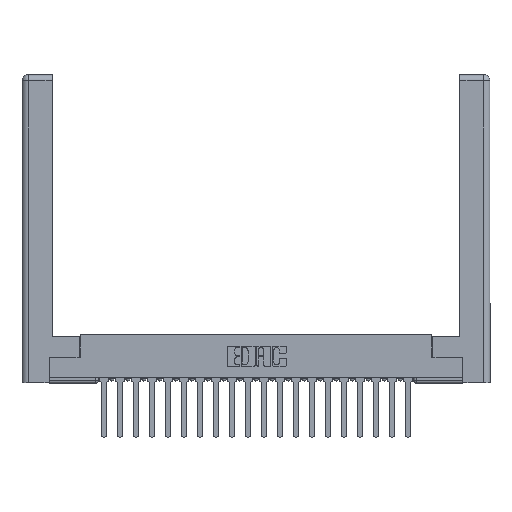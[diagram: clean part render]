
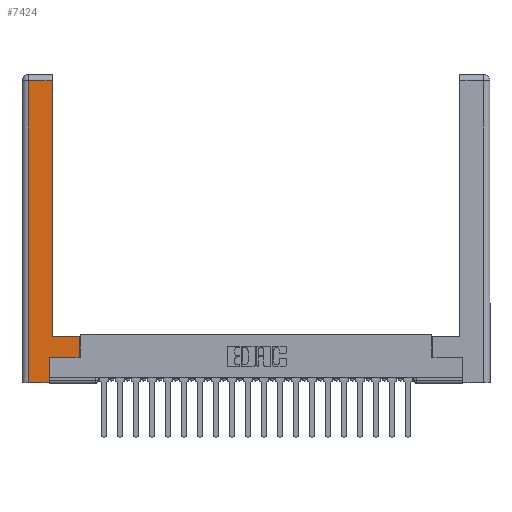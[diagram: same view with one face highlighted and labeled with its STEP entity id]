
A CAD part, top view. The second image highlights one B-rep face of the part: STEP entity #7424.
In plain terms, the highlighted planar face has unit normal (0, 0, 1).
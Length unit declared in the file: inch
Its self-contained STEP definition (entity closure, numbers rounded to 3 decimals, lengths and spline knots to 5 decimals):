
#573 = EDGE_CURVE ( 'NONE', #22322, #12661, #9282, .T. ) ;
#1147 = CARTESIAN_POINT ( 'NONE',  ( 0.0615, 2.94, 0. ) ) ;
#1283 = DIRECTION ( 'NONE',  ( -1., 0., 0. ) ) ;
#1405 = ORIENTED_EDGE ( 'NONE', *, *, #15285, .T. ) ;
#1590 = ORIENTED_EDGE ( 'NONE', *, *, #15119, .T. ) ;
#1652 = VERTEX_POINT ( 'NONE', #21168 ) ;
#1779 = AXIS2_PLACEMENT_3D ( 'NONE', #21097, #19411, #1968 ) ;
#1882 = EDGE_LOOP ( 'NONE', ( #5170, #1590, #4736, #4244, #5856, #15003, #1405, #17423 ) ) ;
#1891 = PLANE ( 'NONE',  #1779 ) ;
#1968 = DIRECTION ( 'NONE',  ( -1., 0., 0. ) ) ;
#2140 = CARTESIAN_POINT ( 'NONE',  ( 0.565, 0.45, 0. ) ) ;
#2605 = DIRECTION ( 'NONE',  ( 1., 0., 0. ) ) ;
#2776 = VECTOR ( 'NONE', #9026, 39.37008 ) ;
#3618 = CARTESIAN_POINT ( 'NONE',  ( 0.565, 0.245, 0. ) ) ;
#4244 = ORIENTED_EDGE ( 'NONE', *, *, #573, .T. ) ;
#4407 = FACE_OUTER_BOUND ( 'NONE', #1882, .T. ) ;
#4505 = VERTEX_POINT ( 'NONE', #8392 ) ;
#4682 = DIRECTION ( 'NONE',  ( 0., 1., 0. ) ) ;
#4711 = EDGE_CURVE ( 'NONE', #1652, #10802, #8016, .T. ) ;
#4736 = ORIENTED_EDGE ( 'NONE', *, *, #14170, .T. ) ;
#4840 = VECTOR ( 'NONE', #1283, 39.37008 ) ;
#5170 = ORIENTED_EDGE ( 'NONE', *, *, #14930, .T. ) ;
#5437 = CARTESIAN_POINT ( 'NONE',  ( 0.0615, 0., 0. ) ) ;
#5856 = ORIENTED_EDGE ( 'NONE', *, *, #10241, .T. ) ;
#6187 = CARTESIAN_POINT ( 'NONE',  ( 0.295, 0.45, 0. ) ) ;
#6730 = CARTESIAN_POINT ( 'NONE',  ( 0.565, 0.245, 0. ) ) ;
#7178 = VECTOR ( 'NONE', #12036, 39.37008 ) ;
#7244 = LINE ( 'NONE', #22209, #4840 ) ;
#7424 = ADVANCED_FACE ( 'NONE', ( #4407 ), #1891, .F. ) ;
#7586 = LINE ( 'NONE', #21042, #19797 ) ;
#7825 = CARTESIAN_POINT ( 'NONE',  ( 0.265, 0., 0. ) ) ;
#8016 = LINE ( 'NONE', #6730, #7178 ) ;
#8392 = CARTESIAN_POINT ( 'NONE',  ( 0.565, 0.45, 0. ) ) ;
#8519 = VERTEX_POINT ( 'NONE', #6187 ) ;
#9026 = DIRECTION ( 'NONE',  ( 0., -1., 0. ) ) ;
#9282 = LINE ( 'NONE', #7825, #16606 ) ;
#10241 = EDGE_CURVE ( 'NONE', #12661, #1652, #11824, .T. ) ;
#10617 = DIRECTION ( 'NONE',  ( -1., 0., 0. ) ) ;
#10802 = VERTEX_POINT ( 'NONE', #3618 ) ;
#11558 = CARTESIAN_POINT ( 'NONE',  ( 0.295, 3., 0. ) ) ;
#11824 = LINE ( 'NONE', #13194, #20284 ) ;
#11925 = LINE ( 'NONE', #11558, #21466 ) ;
#12036 = DIRECTION ( 'NONE',  ( 1., 0., 0. ) ) ;
#12343 = CARTESIAN_POINT ( 'NONE',  ( 0.0615, 0., 0. ) ) ;
#12661 = VERTEX_POINT ( 'NONE', #18261 ) ;
#13194 = CARTESIAN_POINT ( 'NONE',  ( 0.265, 0.245, 0. ) ) ;
#14005 = VERTEX_POINT ( 'NONE', #1147 ) ;
#14079 = VECTOR ( 'NONE', #19350, 39.37008 ) ;
#14170 = EDGE_CURVE ( 'NONE', #14005, #22322, #20396, .T. ) ;
#14930 = EDGE_CURVE ( 'NONE', #8519, #19304, #11925, .T. ) ;
#15003 = ORIENTED_EDGE ( 'NONE', *, *, #4711, .T. ) ;
#15119 = EDGE_CURVE ( 'NONE', #19304, #14005, #7586, .T. ) ;
#15285 = EDGE_CURVE ( 'NONE', #10802, #4505, #18694, .T. ) ;
#16144 = EDGE_CURVE ( 'NONE', #4505, #8519, #7244, .T. ) ;
#16606 = VECTOR ( 'NONE', #2605, 39.37008 ) ;
#17110 = CARTESIAN_POINT ( 'NONE',  ( 0.295, 2.94, 0. ) ) ;
#17423 = ORIENTED_EDGE ( 'NONE', *, *, #16144, .T. ) ;
#18261 = CARTESIAN_POINT ( 'NONE',  ( 0.265, 0., 0. ) ) ;
#18694 = LINE ( 'NONE', #2140, #14079 ) ;
#19304 = VERTEX_POINT ( 'NONE', #17110 ) ;
#19350 = DIRECTION ( 'NONE',  ( 0., 1., 0. ) ) ;
#19411 = DIRECTION ( 'NONE',  ( 0., 0., -1. ) ) ;
#19797 = VECTOR ( 'NONE', #10617, 39.37008 ) ;
#20284 = VECTOR ( 'NONE', #21928, 39.37008 ) ;
#20396 = LINE ( 'NONE', #12343, #2776 ) ;
#21042 = CARTESIAN_POINT ( 'NONE',  ( 0.0615, 2.94, 0. ) ) ;
#21097 = CARTESIAN_POINT ( 'NONE',  ( 0., 0., 0. ) ) ;
#21168 = CARTESIAN_POINT ( 'NONE',  ( 0.265, 0.245, 0. ) ) ;
#21466 = VECTOR ( 'NONE', #4682, 39.37008 ) ;
#21928 = DIRECTION ( 'NONE',  ( 0., 1., 0. ) ) ;
#22209 = CARTESIAN_POINT ( 'NONE',  ( 0.295, 0.45, 0. ) ) ;
#22322 = VERTEX_POINT ( 'NONE', #5437 ) ;
